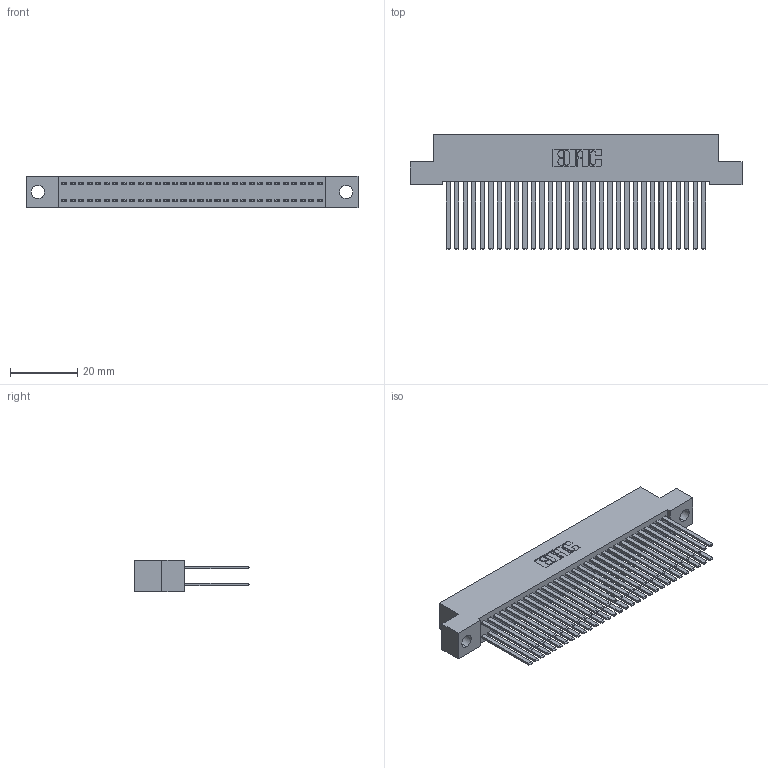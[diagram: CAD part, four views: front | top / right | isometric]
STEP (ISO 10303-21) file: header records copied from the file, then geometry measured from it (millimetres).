
FILE_DESCRIPTION (( 'STEP AP203' ), '1' );
FILE_NAME ('342-062-544-204.STEP', '2018-08-13T06:51:20', ( '' ), ( '' ), 'SwSTEP 2.0', 'SolidWorks 2016', '' );
FILE_SCHEMA (( 'CONFIG_CONTROL_DESIGN' ));
Length unit declared in the file: inch
Products named in the file (3): 342 Part_.156 TH; 345-292-001_345-293-144; 342-062-544-204
Assembly tree (63 placements, depth 2):
  342-062-544-204
    342 Part_.156 TH
    345-292-001_345-293-144  x62
Bounding box: 99.06 x 34.3 x 9.4 mm (x, y, z)
Volume: 9630.6 mm3; surface area: 17636.2 mm2
Topology: 63 solids, 63 shells, 2962 faces, 8793 edges, 5778 vertices
Faces by surface type: plane 2050, cylinder 912
Entity records: 21053 total; most frequent: CARTESIAN_POINT 3498, ORIENTED_EDGE 3434, DIRECTION 3005, EDGE_CURVE 1717, VECTOR 1593, LINE 1593, VERTEX_POINT 1142, AXIS2_PLACEMENT_3D 706
